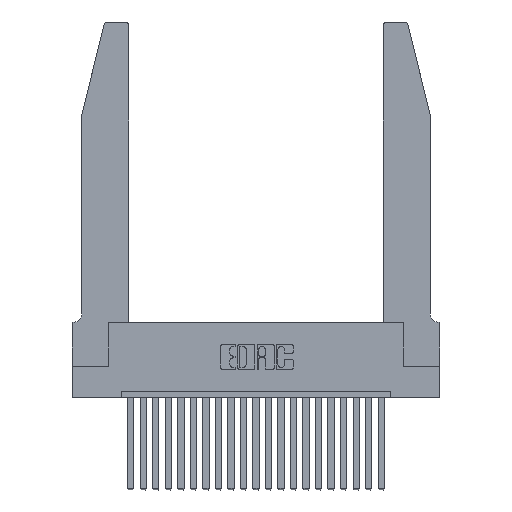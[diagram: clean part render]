
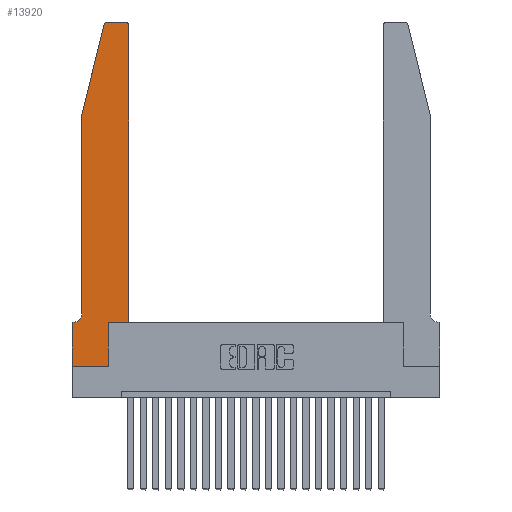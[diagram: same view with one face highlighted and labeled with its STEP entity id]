
A CAD part, top view. The second image highlights one B-rep face of the part: STEP entity #13920.
In plain terms, the highlighted planar face has unit normal (0, 0, 1).
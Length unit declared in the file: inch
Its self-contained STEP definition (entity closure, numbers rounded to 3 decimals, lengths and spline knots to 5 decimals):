
#103 = ORIENTED_EDGE ( 'NONE', *, *, #123, .T. ) ;
#123 = EDGE_CURVE ( 'NONE', #10360, #5144, #16497, .T. ) ;
#398 = DIRECTION ( 'NONE',  ( -1., 0., 0. ) ) ;
#532 = LINE ( 'NONE', #4974, #2816 ) ;
#1048 = VERTEX_POINT ( 'NONE', #1859 ) ;
#1135 = EDGE_CURVE ( 'NONE', #17662, #11803, #4144, .T. ) ;
#1719 = CARTESIAN_POINT ( 'NONE',  ( 0.4505, 0.35, 0.37 ) ) ;
#1859 = CARTESIAN_POINT ( 'NONE',  ( 0.25487, 2.72718, 0.37 ) ) ;
#2451 = CARTESIAN_POINT ( 'NONE',  ( 0.4205, 2.72, 0.37 ) ) ;
#2566 = ORIENTED_EDGE ( 'NONE', *, *, #22178, .T. ) ;
#2649 = CARTESIAN_POINT ( 'NONE',  ( 0.4505, 0.35, 0.37 ) ) ;
#2650 = DIRECTION ( 'NONE',  ( 0., 0., 1. ) ) ;
#2711 = VECTOR ( 'NONE', #3056, 39.37008 ) ;
#2760 = VECTOR ( 'NONE', #6294, 39.37008 ) ;
#2806 = DIRECTION ( 'NONE',  ( 1., 0., 0. ) ) ;
#2816 = VECTOR ( 'NONE', #19278, 39.37008 ) ;
#2874 = VERTEX_POINT ( 'NONE', #9319 ) ;
#2966 = CARTESIAN_POINT ( 'NONE',  ( 0.2865, 0., 0.37 ) ) ;
#3025 = ORIENTED_EDGE ( 'NONE', *, *, #17478, .T. ) ;
#3027 = ORIENTED_EDGE ( 'NONE', *, *, #5166, .T. ) ;
#3056 = DIRECTION ( 'NONE',  ( 0., 1., 0. ) ) ;
#3166 = EDGE_CURVE ( 'NONE', #19664, #22912, #15575, .T. ) ;
#3326 = CARTESIAN_POINT ( 'NONE',  ( 0., 0.35, 0.37 ) ) ;
#3413 = PLANE ( 'NONE',  #19392 ) ;
#3710 = LINE ( 'NONE', #18473, #22710 ) ;
#3948 = ORIENTED_EDGE ( 'NONE', *, *, #15965, .T. ) ;
#4136 = VERTEX_POINT ( 'NONE', #18719 ) ;
#4144 = LINE ( 'NONE', #9079, #6956 ) ;
#4210 = CARTESIAN_POINT ( 'NONE',  ( 0.2865, 0.35, 0.37 ) ) ;
#4778 = CARTESIAN_POINT ( 'NONE',  ( 0., 0., 0.37 ) ) ;
#4910 = CARTESIAN_POINT ( 'NONE',  ( 0.0055, 0.35, 0.37 ) ) ;
#4974 = CARTESIAN_POINT ( 'NONE',  ( 0., 0., 0.37 ) ) ;
#5144 = VERTEX_POINT ( 'NONE', #14939 ) ;
#5166 = EDGE_CURVE ( 'NONE', #1048, #17662, #3710, .T. ) ;
#6015 = CARTESIAN_POINT ( 'NONE',  ( 0.2865, 0.35, 0.37 ) ) ;
#6018 = DIRECTION ( 'NONE',  ( -1., 0., 0. ) ) ;
#6211 = CARTESIAN_POINT ( 'NONE',  ( 0.2605, 2.75, 0.37 ) ) ;
#6294 = DIRECTION ( 'NONE',  ( -1., 0., 0. ) ) ;
#6757 = EDGE_CURVE ( 'NONE', #22912, #21778, #10512, .T. ) ;
#6956 = VECTOR ( 'NONE', #20096, 39.37008 ) ;
#7143 = LINE ( 'NONE', #4778, #10449 ) ;
#7946 = DIRECTION ( 'NONE',  ( 0., 0., 1. ) ) ;
#8313 = CARTESIAN_POINT ( 'NONE',  ( 0.4505, 0.35, 0.37 ) ) ;
#8417 = VECTOR ( 'NONE', #398, 39.37008 ) ;
#8462 = VECTOR ( 'NONE', #9485, 39.37008 ) ;
#8730 = DIRECTION ( 'NONE',  ( 1., 0., 0. ) ) ;
#9079 = CARTESIAN_POINT ( 'NONE',  ( 0.0755, 2., 0.37 ) ) ;
#9172 = LINE ( 'NONE', #6015, #14450 ) ;
#9319 = CARTESIAN_POINT ( 'NONE',  ( 0., 0., 0.37 ) ) ;
#9485 = DIRECTION ( 'NONE',  ( 1., 0., 0. ) ) ;
#9844 = DIRECTION ( 'NONE',  ( 0., -1., 0. ) ) ;
#10360 = VERTEX_POINT ( 'NONE', #4910 ) ;
#10449 = VECTOR ( 'NONE', #9844, 39.37008 ) ;
#10512 = CIRCLE ( 'NONE', #12819, 0.03 ) ;
#10790 = CARTESIAN_POINT ( 'NONE',  ( 0.4205, 2.75, 0.37 ) ) ;
#10868 = EDGE_CURVE ( 'NONE', #2874, #12787, #532, .T. ) ;
#10876 = ORIENTED_EDGE ( 'NONE', *, *, #12467, .T. ) ;
#11276 = DIRECTION ( 'NONE',  ( -0.239, -0.971, 0. ) ) ;
#11803 = VERTEX_POINT ( 'NONE', #12731 ) ;
#11846 = CIRCLE ( 'NONE', #16130, 0.03 ) ;
#11908 = AXIS2_PLACEMENT_3D ( 'NONE', #18268, #13165, #6018 ) ;
#12467 = EDGE_CURVE ( 'NONE', #12787, #20784, #9172, .T. ) ;
#12731 = CARTESIAN_POINT ( 'NONE',  ( 0.0755, 0.42, 0.37 ) ) ;
#12787 = VERTEX_POINT ( 'NONE', #2966 ) ;
#12819 = AXIS2_PLACEMENT_3D ( 'NONE', #2451, #7946, #15105 ) ;
#13165 = DIRECTION ( 'NONE',  ( 0., 0., -1. ) ) ;
#13269 = CARTESIAN_POINT ( 'NONE',  ( 0.284, 2.72, 0.37 ) ) ;
#13920 = ADVANCED_FACE ( 'NONE', ( #20663 ), #3413, .T. ) ;
#14450 = VECTOR ( 'NONE', #15120, 39.37008 ) ;
#14699 = CIRCLE ( 'NONE', #11908, 0.07 ) ;
#14939 = CARTESIAN_POINT ( 'NONE',  ( 0., 0.35, 0.37 ) ) ;
#15105 = DIRECTION ( 'NONE',  ( 1., 0., 0. ) ) ;
#15120 = DIRECTION ( 'NONE',  ( 0., 1., 0. ) ) ;
#15575 = LINE ( 'NONE', #8313, #2711 ) ;
#15965 = EDGE_CURVE ( 'NONE', #11803, #10360, #14699, .T. ) ;
#16130 = AXIS2_PLACEMENT_3D ( 'NONE', #13269, #2650, #2806 ) ;
#16497 = LINE ( 'NONE', #16709, #8417 ) ;
#16709 = CARTESIAN_POINT ( 'NONE',  ( 0.0755, 0.35, 0.37 ) ) ;
#17065 = EDGE_CURVE ( 'NONE', #5144, #2874, #7143, .T. ) ;
#17098 = ORIENTED_EDGE ( 'NONE', *, *, #10868, .T. ) ;
#17478 = EDGE_CURVE ( 'NONE', #4136, #1048, #11846, .T. ) ;
#17662 = VERTEX_POINT ( 'NONE', #19465 ) ;
#17723 = CARTESIAN_POINT ( 'NONE',  ( 0.4505, 2.72, 0.37 ) ) ;
#17824 = ORIENTED_EDGE ( 'NONE', *, *, #17065, .T. ) ;
#17945 = DIRECTION ( 'NONE',  ( 0., 0., 1. ) ) ;
#18242 = EDGE_LOOP ( 'NONE', ( #2566, #3025, #3027, #21418, #3948, #103, #17824, #17098, #10876, #19951, #20554, #20115 ) ) ;
#18268 = CARTESIAN_POINT ( 'NONE',  ( 0.0055, 0.42, 0.37 ) ) ;
#18473 = CARTESIAN_POINT ( 'NONE',  ( 0.0755, 2., 0.37 ) ) ;
#18548 = EDGE_CURVE ( 'NONE', #20784, #19664, #18804, .T. ) ;
#18719 = CARTESIAN_POINT ( 'NONE',  ( 0.284, 2.75, 0.37 ) ) ;
#18804 = LINE ( 'NONE', #1719, #8462 ) ;
#19278 = DIRECTION ( 'NONE',  ( 1., 0., 0. ) ) ;
#19392 = AXIS2_PLACEMENT_3D ( 'NONE', #3326, #17945, #8730 ) ;
#19465 = CARTESIAN_POINT ( 'NONE',  ( 0.0755, 2., 0.37 ) ) ;
#19664 = VERTEX_POINT ( 'NONE', #2649 ) ;
#19951 = ORIENTED_EDGE ( 'NONE', *, *, #18548, .T. ) ;
#20096 = DIRECTION ( 'NONE',  ( 0., -1., 0. ) ) ;
#20104 = LINE ( 'NONE', #6211, #2760 ) ;
#20115 = ORIENTED_EDGE ( 'NONE', *, *, #6757, .T. ) ;
#20554 = ORIENTED_EDGE ( 'NONE', *, *, #3166, .T. ) ;
#20663 = FACE_OUTER_BOUND ( 'NONE', #18242, .T. ) ;
#20784 = VERTEX_POINT ( 'NONE', #4210 ) ;
#21418 = ORIENTED_EDGE ( 'NONE', *, *, #1135, .T. ) ;
#21778 = VERTEX_POINT ( 'NONE', #10790 ) ;
#22178 = EDGE_CURVE ( 'NONE', #21778, #4136, #20104, .T. ) ;
#22710 = VECTOR ( 'NONE', #11276, 39.37008 ) ;
#22912 = VERTEX_POINT ( 'NONE', #17723 ) ;
